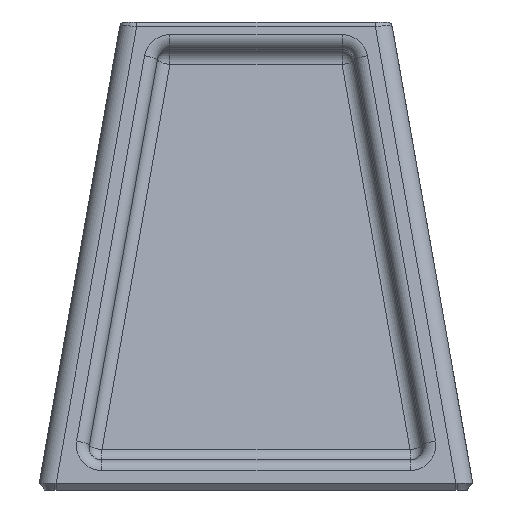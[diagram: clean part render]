
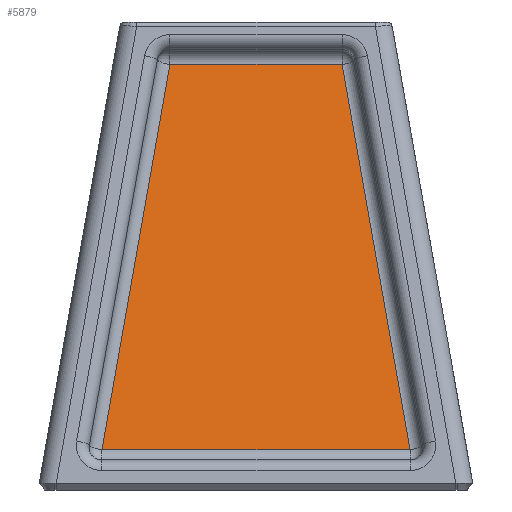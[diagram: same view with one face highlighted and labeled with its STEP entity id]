
A CAD part, left-side view. The second image highlights one B-rep face of the part: STEP entity #5879.
In plain terms, the highlighted planar face has unit normal (-0.985, 0, 0.174).
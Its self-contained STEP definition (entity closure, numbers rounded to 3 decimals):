
#626=PLANE('',#6263);
#919=FACE_OUTER_BOUND('',#1281,.T.);
#1281=EDGE_LOOP('',(#5170,#5171,#5172,#5173));
#1729=LINE('',#11805,#2155);
#1730=LINE('',#11807,#2156);
#1731=LINE('',#11809,#2157);
#1732=LINE('',#11810,#2158);
#2155=VECTOR('',#7375,10.);
#2156=VECTOR('',#7376,10.);
#2157=VECTOR('',#7377,10.);
#2158=VECTOR('',#7378,10.);
#2820=VERTEX_POINT('',#11803);
#2821=VERTEX_POINT('',#11804);
#2822=VERTEX_POINT('',#11806);
#2823=VERTEX_POINT('',#11808);
#3633=EDGE_CURVE('',#2820,#2821,#1729,.T.);
#3634=EDGE_CURVE('',#2822,#2820,#1730,.T.);
#3635=EDGE_CURVE('',#2823,#2822,#1731,.T.);
#3636=EDGE_CURVE('',#2821,#2823,#1732,.T.);
#5170=ORIENTED_EDGE('',*,*,#3633,.F.);
#5171=ORIENTED_EDGE('',*,*,#3634,.F.);
#5172=ORIENTED_EDGE('',*,*,#3635,.F.);
#5173=ORIENTED_EDGE('',*,*,#3636,.F.);
#5879=ADVANCED_FACE('',(#919),#626,.F.);
#6263=AXIS2_PLACEMENT_3D('',#11802,#7373,#7374);
#7373=DIRECTION('center_axis',(0.985,0.,-0.174));
#7374=DIRECTION('ref_axis',(-0.174,0.,-0.985));
#7375=DIRECTION('',(-0.171,-0.171,-0.97));
#7376=DIRECTION('',(0.,-1.,0.));
#7377=DIRECTION('',(0.171,-0.171,0.97));
#7378=DIRECTION('',(0.,1.,0.));
#11802=CARTESIAN_POINT('Origin',(-53.79,0.,
-1.827));
#11803=CARTESIAN_POINT('',(-49.827,-10.044,20.647));
#11804=CARTESIAN_POINT('',(-57.753,-17.97,-24.301));
#11805=CARTESIAN_POINT('',(-51.495,-11.713,11.185));
#11806=CARTESIAN_POINT('',(-49.827,10.044,20.647));
#11807=CARTESIAN_POINT('',(-49.827,5.653,20.647));
#11808=CARTESIAN_POINT('',(-57.753,17.97,-24.301));
#11809=CARTESIAN_POINT('',(-55.719,15.936,-12.767));
#11810=CARTESIAN_POINT('',(-57.753,-9.877,-24.301));
